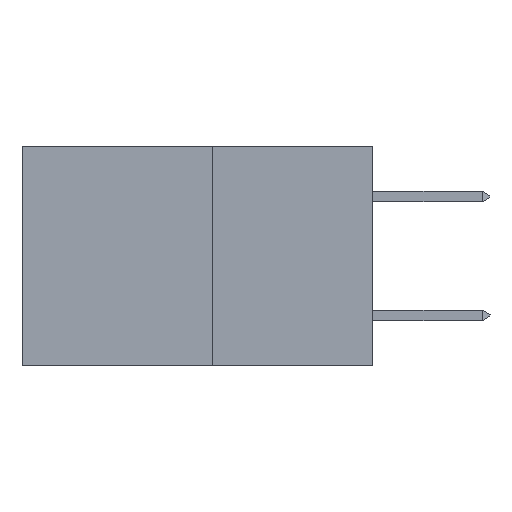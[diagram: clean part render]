
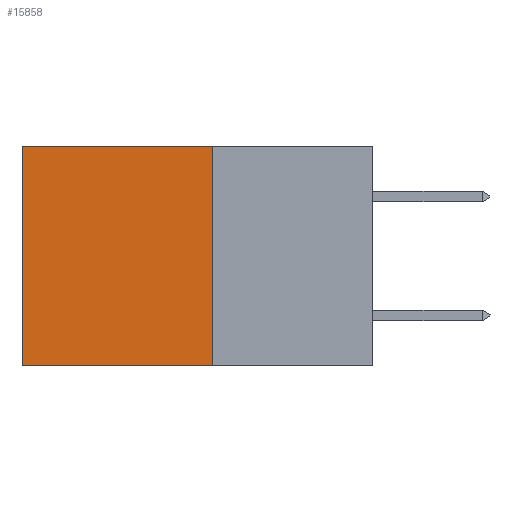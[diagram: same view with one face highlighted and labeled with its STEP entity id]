
A CAD part, left-side view. The second image highlights one B-rep face of the part: STEP entity #15858.
In plain terms, the highlighted planar face has unit normal (-1, 0, 0).
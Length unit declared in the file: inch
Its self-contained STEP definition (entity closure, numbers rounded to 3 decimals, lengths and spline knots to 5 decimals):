
#137 = CARTESIAN_POINT ( 'NONE',  ( 0.277, 0.59, -0.37 ) ) ;
#499 = EDGE_CURVE ( 'NONE', #19537, #12177, #21340, .T. ) ;
#1495 = PLANE ( 'NONE',  #18693 ) ;
#1821 = ORIENTED_EDGE ( 'NONE', *, *, #23926, .T. ) ;
#2406 = LINE ( 'NONE', #7379, #23063 ) ;
#2588 = DIRECTION ( 'NONE',  ( 0., 1., 0. ) ) ;
#3578 = DIRECTION ( 'NONE',  ( 1., 0., 0. ) ) ;
#5287 = DIRECTION ( 'NONE',  ( 0., 0., -1. ) ) ;
#5705 = VECTOR ( 'NONE', #8578, 39.37008 ) ;
#6078 = CARTESIAN_POINT ( 'NONE',  ( 0.277, 0.27, -0.37 ) ) ;
#7102 = VERTEX_POINT ( 'NONE', #16700 ) ;
#7379 = CARTESIAN_POINT ( 'NONE',  ( 0.277, 0.27, -0.37 ) ) ;
#7686 = VERTEX_POINT ( 'NONE', #6078 ) ;
#8540 = EDGE_CURVE ( 'NONE', #7686, #12177, #22164, .T. ) ;
#8578 = DIRECTION ( 'NONE',  ( 0., 1., 0. ) ) ;
#10761 = EDGE_CURVE ( 'NONE', #7102, #7686, #2406, .T. ) ;
#11245 = LINE ( 'NONE', #14977, #16090 ) ;
#11349 = DIRECTION ( 'NONE',  ( 0., 0., -1. ) ) ;
#12177 = VERTEX_POINT ( 'NONE', #19785 ) ;
#13899 = CARTESIAN_POINT ( 'NONE',  ( 0.277, 0.27, -0.37 ) ) ;
#14455 = ORIENTED_EDGE ( 'NONE', *, *, #499, .T. ) ;
#14977 = CARTESIAN_POINT ( 'NONE',  ( 0.277, 0.27, 0. ) ) ;
#15858 = ADVANCED_FACE ( 'NONE', ( #21787 ), #1495, .F. ) ;
#16090 = VECTOR ( 'NONE', #2588, 39.37008 ) ;
#16700 = CARTESIAN_POINT ( 'NONE',  ( 0.277, 0.27, 0. ) ) ;
#17591 = EDGE_LOOP ( 'NONE', ( #14455, #21849, #23156, #1821 ) ) ;
#18065 = DIRECTION ( 'NONE',  ( 0., 0., -1. ) ) ;
#18693 = AXIS2_PLACEMENT_3D ( 'NONE', #13899, #3578, #18065 ) ;
#19537 = VERTEX_POINT ( 'NONE', #23629 ) ;
#19785 = CARTESIAN_POINT ( 'NONE',  ( 0.277, 0.59, -0.37 ) ) ;
#20691 = VECTOR ( 'NONE', #11349, 39.37008 ) ;
#21340 = LINE ( 'NONE', #137, #20691 ) ;
#21787 = FACE_OUTER_BOUND ( 'NONE', #17591, .T. ) ;
#21849 = ORIENTED_EDGE ( 'NONE', *, *, #8540, .F. ) ;
#22164 = LINE ( 'NONE', #25035, #5705 ) ;
#23063 = VECTOR ( 'NONE', #5287, 39.37008 ) ;
#23156 = ORIENTED_EDGE ( 'NONE', *, *, #10761, .F. ) ;
#23629 = CARTESIAN_POINT ( 'NONE',  ( 0.277, 0.59, 0. ) ) ;
#23926 = EDGE_CURVE ( 'NONE', #7102, #19537, #11245, .T. ) ;
#25035 = CARTESIAN_POINT ( 'NONE',  ( 0.277, 0.27, -0.37 ) ) ;
